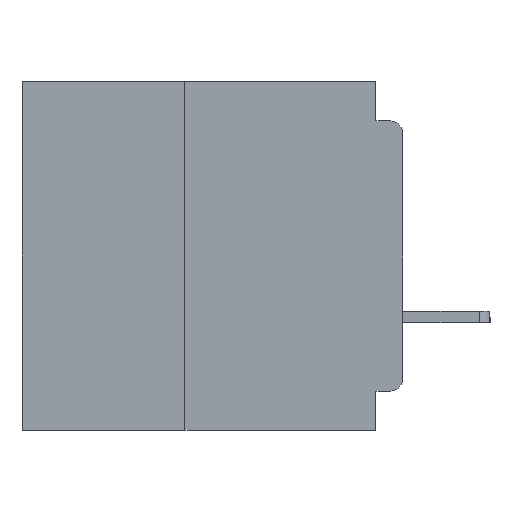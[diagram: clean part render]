
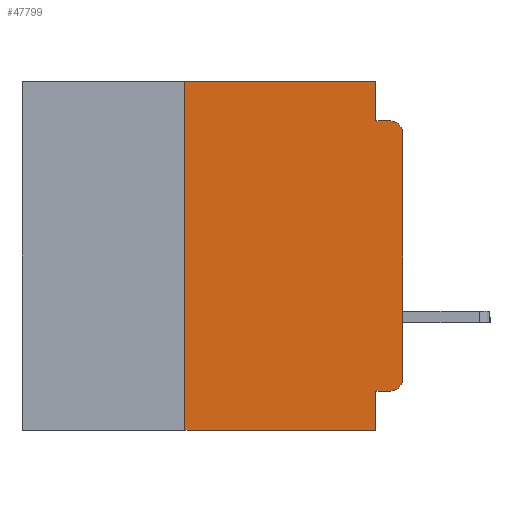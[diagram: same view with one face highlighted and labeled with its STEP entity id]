
A CAD part, left-side view. The second image highlights one B-rep face of the part: STEP entity #47799.
In plain terms, the highlighted planar face has unit normal (-1, 0, 0).
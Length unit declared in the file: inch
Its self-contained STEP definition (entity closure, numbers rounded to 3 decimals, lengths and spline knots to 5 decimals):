
#55 = LINE ( 'NONE', #2819, #38987 ) ;
#533 = DIRECTION ( 'NONE',  ( 0., -1., 0. ) ) ;
#842 = ORIENTED_EDGE ( 'NONE', *, *, #64968, .F. ) ;
#2635 = FACE_OUTER_BOUND ( 'NONE', #66592, .T. ) ;
#2672 = DIRECTION ( 'NONE',  ( 0., 0., -1. ) ) ;
#2819 = CARTESIAN_POINT ( 'NONE',  ( 0., 0., 0. ) ) ;
#4344 = VERTEX_POINT ( 'NONE', #58035 ) ;
#4453 = LINE ( 'NONE', #59670, #30960 ) ;
#6229 = CARTESIAN_POINT ( 'NONE',  ( 0., 0.031, 0. ) ) ;
#6849 = CARTESIAN_POINT ( 'NONE',  ( 0., 0.25, -0.4 ) ) ;
#7090 = DIRECTION ( 'NONE',  ( 0., 0., -1. ) ) ;
#7309 = DIRECTION ( 'NONE',  ( 0., 0., 1. ) ) ;
#8128 = DIRECTION ( 'NONE',  ( 0., 0., 1. ) ) ;
#8790 = LINE ( 'NONE', #6849, #63288 ) ;
#10806 = CARTESIAN_POINT ( 'NONE',  ( 0., 0., -0.355 ) ) ;
#12597 = VERTEX_POINT ( 'NONE', #48091 ) ;
#13207 = ORIENTED_EDGE ( 'NONE', *, *, #60497, .F. ) ;
#13635 = ORIENTED_EDGE ( 'NONE', *, *, #61126, .T. ) ;
#14557 = CARTESIAN_POINT ( 'NONE',  ( 0., 0.25, -0.4 ) ) ;
#14932 = VERTEX_POINT ( 'NONE', #57815 ) ;
#15358 = VECTOR ( 'NONE', #533, 39.37008 ) ;
#17448 = ORIENTED_EDGE ( 'NONE', *, *, #50433, .F. ) ;
#18741 = VERTEX_POINT ( 'NONE', #59543 ) ;
#20197 = ORIENTED_EDGE ( 'NONE', *, *, #46265, .T. ) ;
#21227 = LINE ( 'NONE', #44105, #61661 ) ;
#21447 = DIRECTION ( 'NONE',  ( 0., 1., 0. ) ) ;
#22280 = CARTESIAN_POINT ( 'NONE',  ( 0., 0.015, -0.355 ) ) ;
#22731 = CARTESIAN_POINT ( 'NONE',  ( 0., 0.015, -0.34 ) ) ;
#24286 = CIRCLE ( 'NONE', #37487, 0.015 ) ;
#24432 = CARTESIAN_POINT ( 'NONE',  ( 0., 0.015, -0.06 ) ) ;
#24733 = VERTEX_POINT ( 'NONE', #14557 ) ;
#25441 = VERTEX_POINT ( 'NONE', #47546 ) ;
#26040 = AXIS2_PLACEMENT_3D ( 'NONE', #31351, #63097, #31573 ) ;
#27083 = DIRECTION ( 'NONE',  ( 0., -1., 0. ) ) ;
#28052 = DIRECTION ( 'NONE',  ( 0., 0., -1. ) ) ;
#28553 = VECTOR ( 'NONE', #27083, 39.37008 ) ;
#28898 = EDGE_CURVE ( 'NONE', #56365, #18741, #53636, .T. ) ;
#29066 = CARTESIAN_POINT ( 'NONE',  ( 0., 0.031, 0. ) ) ;
#29479 = LINE ( 'NONE', #37552, #15358 ) ;
#29561 = VECTOR ( 'NONE', #21447, 39.37008 ) ;
#29783 = DIRECTION ( 'NONE',  ( 0., 0., -1. ) ) ;
#30960 = VECTOR ( 'NONE', #64872, 39.37008 ) ;
#31351 = CARTESIAN_POINT ( 'NONE',  ( 0., 0.437, 0. ) ) ;
#31369 = CIRCLE ( 'NONE', #51524, 0.015 ) ;
#31573 = DIRECTION ( 'NONE',  ( 0., 0., -1. ) ) ;
#32401 = CARTESIAN_POINT ( 'NONE',  ( 0., 0.437, -0.4 ) ) ;
#34451 = ORIENTED_EDGE ( 'NONE', *, *, #28898, .F. ) ;
#37180 = CARTESIAN_POINT ( 'NONE',  ( 0., 0., -0.34 ) ) ;
#37487 = AXIS2_PLACEMENT_3D ( 'NONE', #22731, #59665, #28052 ) ;
#37552 = CARTESIAN_POINT ( 'NONE',  ( 0., 0., -0.045 ) ) ;
#37891 = CARTESIAN_POINT ( 'NONE',  ( 0., 0.031, -0.355 ) ) ;
#37963 = VECTOR ( 'NONE', #2672, 39.37008 ) ;
#38987 = VECTOR ( 'NONE', #8128, 39.37008 ) ;
#40807 = VERTEX_POINT ( 'NONE', #37891 ) ;
#41729 = PLANE ( 'NONE',  #26040 ) ;
#41969 = EDGE_CURVE ( 'NONE', #24733, #4344, #8790, .T. ) ;
#42888 = ORIENTED_EDGE ( 'NONE', *, *, #67184, .T. ) ;
#43432 = VERTEX_POINT ( 'NONE', #37180 ) ;
#44105 = CARTESIAN_POINT ( 'NONE',  ( 0., 0.031, -0.4 ) ) ;
#44246 = LINE ( 'NONE', #32401, #28553 ) ;
#46265 = EDGE_CURVE ( 'NONE', #47937, #43432, #24286, .T. ) ;
#47546 = CARTESIAN_POINT ( 'NONE',  ( 0., 0.015, -0.045 ) ) ;
#47799 = ADVANCED_FACE ( 'NONE', ( #2635 ), #41729, .F. ) ;
#47937 = VERTEX_POINT ( 'NONE', #22280 ) ;
#48091 = CARTESIAN_POINT ( 'NONE',  ( 0., 0.031, -0.4 ) ) ;
#50433 = EDGE_CURVE ( 'NONE', #47937, #40807, #57571, .T. ) ;
#50597 = EDGE_CURVE ( 'NONE', #40807, #12597, #21227, .T. ) ;
#51524 = AXIS2_PLACEMENT_3D ( 'NONE', #24432, #61340, #29783 ) ;
#52231 = ORIENTED_EDGE ( 'NONE', *, *, #41969, .F. ) ;
#53636 = LINE ( 'NONE', #29066, #37963 ) ;
#56365 = VERTEX_POINT ( 'NONE', #6229 ) ;
#57571 = LINE ( 'NONE', #10806, #29561 ) ;
#57815 = CARTESIAN_POINT ( 'NONE',  ( 0., 0., -0.06 ) ) ;
#58035 = CARTESIAN_POINT ( 'NONE',  ( 0., 0.25, 0. ) ) ;
#59543 = CARTESIAN_POINT ( 'NONE',  ( 0., 0.031, -0.045 ) ) ;
#59665 = DIRECTION ( 'NONE',  ( -1., 0., 0. ) ) ;
#59670 = CARTESIAN_POINT ( 'NONE',  ( 0., 0.437, 0. ) ) ;
#60497 = EDGE_CURVE ( 'NONE', #18741, #25441, #29479, .T. ) ;
#60722 = ORIENTED_EDGE ( 'NONE', *, *, #68446, .T. ) ;
#61064 = ORIENTED_EDGE ( 'NONE', *, *, #50597, .F. ) ;
#61126 = EDGE_CURVE ( 'NONE', #24733, #12597, #44246, .T. ) ;
#61340 = DIRECTION ( 'NONE',  ( -1., 0., 0. ) ) ;
#61661 = VECTOR ( 'NONE', #7090, 39.37008 ) ;
#63097 = DIRECTION ( 'NONE',  ( 1., 0., 0. ) ) ;
#63288 = VECTOR ( 'NONE', #7309, 39.37008 ) ;
#64872 = DIRECTION ( 'NONE',  ( 0., -1., 0. ) ) ;
#64968 = EDGE_CURVE ( 'NONE', #4344, #56365, #4453, .T. ) ;
#66592 = EDGE_LOOP ( 'NONE', ( #42888, #60722, #13207, #34451, #842, #52231, #13635, #61064, #17448, #20197 ) ) ;
#67184 = EDGE_CURVE ( 'NONE', #43432, #14932, #55, .T. ) ;
#68446 = EDGE_CURVE ( 'NONE', #14932, #25441, #31369, .T. ) ;
